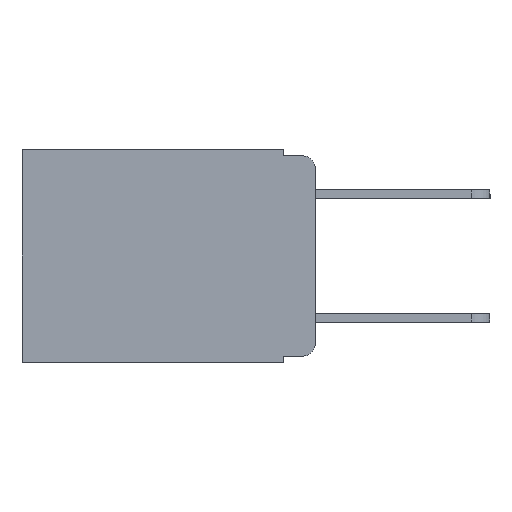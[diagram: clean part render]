
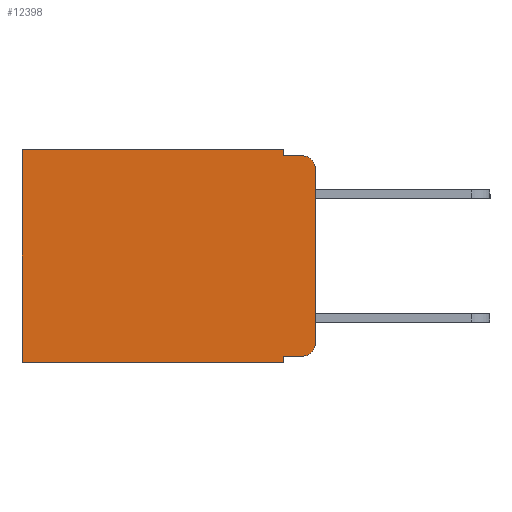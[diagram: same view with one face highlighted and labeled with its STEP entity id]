
A CAD part, left-side view. The second image highlights one B-rep face of the part: STEP entity #12398.
In plain terms, the highlighted planar face has unit normal (-1, 0, 0).
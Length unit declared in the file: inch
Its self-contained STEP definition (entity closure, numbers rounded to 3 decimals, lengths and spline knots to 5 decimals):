
#385 = ORIENTED_EDGE ( 'NONE', *, *, #9014, .F. ) ;
#424 = EDGE_CURVE ( 'NONE', #17453, #2747, #10296, .T. ) ;
#955 = ORIENTED_EDGE ( 'NONE', *, *, #424, .T. ) ;
#1090 = CIRCLE ( 'NONE', #9898, 0.02 ) ;
#1267 = ORIENTED_EDGE ( 'NONE', *, *, #13289, .T. ) ;
#1404 = CARTESIAN_POINT ( 'NONE',  ( 0.298, 0., -0.343 ) ) ;
#1830 = AXIS2_PLACEMENT_3D ( 'NONE', #9392, #3916, #16649 ) ;
#1845 = CARTESIAN_POINT ( 'NONE',  ( 0.298, 0.051, -0.333 ) ) ;
#2024 = CARTESIAN_POINT ( 'NONE',  ( 0.298, 0.02, -0.313 ) ) ;
#2095 = VECTOR ( 'NONE', #18577, 39.37008 ) ;
#2640 = FACE_OUTER_BOUND ( 'NONE', #6021, .T. ) ;
#2747 = VERTEX_POINT ( 'NONE', #14644 ) ;
#3060 = ORIENTED_EDGE ( 'NONE', *, *, #16539, .T. ) ;
#3456 = EDGE_CURVE ( 'NONE', #6508, #5464, #7482, .T. ) ;
#3916 = DIRECTION ( 'NONE',  ( 1., 0., 0. ) ) ;
#3923 = DIRECTION ( 'NONE',  ( 0., 0., -1. ) ) ;
#4153 = DIRECTION ( 'NONE',  ( 0., -1., 0. ) ) ;
#5259 = CARTESIAN_POINT ( 'NONE',  ( 0.298, 0.02, -0.01 ) ) ;
#5464 = VERTEX_POINT ( 'NONE', #23583 ) ;
#5506 = EDGE_CURVE ( 'NONE', #10501, #12609, #16682, .T. ) ;
#6021 = EDGE_LOOP ( 'NONE', ( #19561, #1267, #21230, #10228, #3060, #955, #385, #8347, #8258, #11509 ) ) ;
#6134 = CARTESIAN_POINT ( 'NONE',  ( 0.298, 0., -0.03 ) ) ;
#6176 = LINE ( 'NONE', #10729, #20030 ) ;
#6177 = CARTESIAN_POINT ( 'NONE',  ( 0.298, 0.473, 0. ) ) ;
#6404 = CARTESIAN_POINT ( 'NONE',  ( 0.298, 0.02, -0.03 ) ) ;
#6508 = VERTEX_POINT ( 'NONE', #6134 ) ;
#7482 = LINE ( 'NONE', #15645, #11097 ) ;
#7708 = DIRECTION ( 'NONE',  ( 0., 0., -1. ) ) ;
#7946 = VERTEX_POINT ( 'NONE', #18668 ) ;
#7990 = CARTESIAN_POINT ( 'NONE',  ( 0.298, 0.051, 0. ) ) ;
#8238 = DIRECTION ( 'NONE',  ( 0., 0., -1. ) ) ;
#8258 = ORIENTED_EDGE ( 'NONE', *, *, #12832, .T. ) ;
#8347 = ORIENTED_EDGE ( 'NONE', *, *, #5506, .F. ) ;
#8455 = EDGE_CURVE ( 'NONE', #7946, #21147, #20206, .T. ) ;
#8539 = CARTESIAN_POINT ( 'NONE',  ( 0.298, 0.02, -0.333 ) ) ;
#9014 = EDGE_CURVE ( 'NONE', #12609, #2747, #16779, .T. ) ;
#9392 = CARTESIAN_POINT ( 'NONE',  ( 0.298, 0., 0. ) ) ;
#9742 = VECTOR ( 'NONE', #7708, 39.37008 ) ;
#9898 = AXIS2_PLACEMENT_3D ( 'NONE', #2024, #14889, #3923 ) ;
#10228 = ORIENTED_EDGE ( 'NONE', *, *, #19326, .F. ) ;
#10296 = LINE ( 'NONE', #16489, #9742 ) ;
#10501 = VERTEX_POINT ( 'NONE', #1845 ) ;
#10699 = CARTESIAN_POINT ( 'NONE',  ( 0.298, 0.051, -0.333 ) ) ;
#10719 = VERTEX_POINT ( 'NONE', #17111 ) ;
#10729 = CARTESIAN_POINT ( 'NONE',  ( 0.298, 0.051, 0. ) ) ;
#11097 = VECTOR ( 'NONE', #20883, 39.37008 ) ;
#11509 = ORIENTED_EDGE ( 'NONE', *, *, #21265, .T. ) ;
#12398 = ADVANCED_FACE ( 'NONE', ( #2640 ), #16576, .F. ) ;
#12510 = LINE ( 'NONE', #19963, #16722 ) ;
#12546 = DIRECTION ( 'NONE',  ( 0., -1., 0. ) ) ;
#12609 = VERTEX_POINT ( 'NONE', #20905 ) ;
#12823 = DIRECTION ( 'NONE',  ( 0., 1., 0. ) ) ;
#12832 = EDGE_CURVE ( 'NONE', #10501, #21608, #20851, .T. ) ;
#13289 = EDGE_CURVE ( 'NONE', #6508, #21147, #16309, .T. ) ;
#14238 = CARTESIAN_POINT ( 'NONE',  ( 0.298, 0.051, -0.01 ) ) ;
#14536 = DIRECTION ( 'NONE',  ( 0., 1., 0. ) ) ;
#14644 = CARTESIAN_POINT ( 'NONE',  ( 0.298, 0.473, -0.343 ) ) ;
#14889 = DIRECTION ( 'NONE',  ( -1., 0., 0. ) ) ;
#15645 = CARTESIAN_POINT ( 'NONE',  ( 0.298, 0., 0. ) ) ;
#16083 = VECTOR ( 'NONE', #12546, 39.37008 ) ;
#16309 = CIRCLE ( 'NONE', #21691, 0.02 ) ;
#16489 = CARTESIAN_POINT ( 'NONE',  ( 0.298, 0.473, 0. ) ) ;
#16539 = EDGE_CURVE ( 'NONE', #10719, #17453, #12510, .T. ) ;
#16576 = PLANE ( 'NONE',  #1830 ) ;
#16649 = DIRECTION ( 'NONE',  ( 0., 0., -1. ) ) ;
#16682 = LINE ( 'NONE', #7990, #2095 ) ;
#16722 = VECTOR ( 'NONE', #14536, 39.37008 ) ;
#16779 = LINE ( 'NONE', #1404, #21026 ) ;
#17111 = CARTESIAN_POINT ( 'NONE',  ( 0.298, 0.051, 0. ) ) ;
#17453 = VERTEX_POINT ( 'NONE', #6177 ) ;
#18577 = DIRECTION ( 'NONE',  ( 0., 0., -1. ) ) ;
#18668 = CARTESIAN_POINT ( 'NONE',  ( 0.298, 0.051, -0.01 ) ) ;
#19053 = DIRECTION ( 'NONE',  ( -1., 0., 0. ) ) ;
#19326 = EDGE_CURVE ( 'NONE', #10719, #7946, #6176, .T. ) ;
#19561 = ORIENTED_EDGE ( 'NONE', *, *, #3456, .F. ) ;
#19647 = VECTOR ( 'NONE', #4153, 39.37008 ) ;
#19963 = CARTESIAN_POINT ( 'NONE',  ( 0.298, 0., 0. ) ) ;
#20030 = VECTOR ( 'NONE', #21543, 39.37008 ) ;
#20206 = LINE ( 'NONE', #14238, #19647 ) ;
#20851 = LINE ( 'NONE', #10699, #16083 ) ;
#20883 = DIRECTION ( 'NONE',  ( 0., 0., -1. ) ) ;
#20905 = CARTESIAN_POINT ( 'NONE',  ( 0.298, 0.051, -0.343 ) ) ;
#21026 = VECTOR ( 'NONE', #12823, 39.37008 ) ;
#21147 = VERTEX_POINT ( 'NONE', #5259 ) ;
#21230 = ORIENTED_EDGE ( 'NONE', *, *, #8455, .F. ) ;
#21265 = EDGE_CURVE ( 'NONE', #21608, #5464, #1090, .T. ) ;
#21543 = DIRECTION ( 'NONE',  ( 0., 0., -1. ) ) ;
#21608 = VERTEX_POINT ( 'NONE', #8539 ) ;
#21691 = AXIS2_PLACEMENT_3D ( 'NONE', #6404, #19053, #8238 ) ;
#23583 = CARTESIAN_POINT ( 'NONE',  ( 0.298, 0., -0.313 ) ) ;
